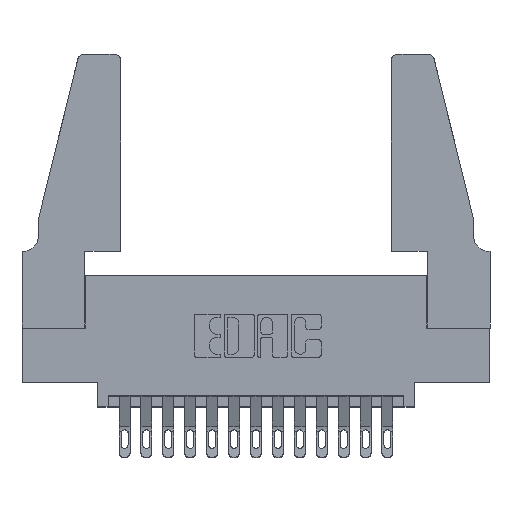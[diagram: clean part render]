
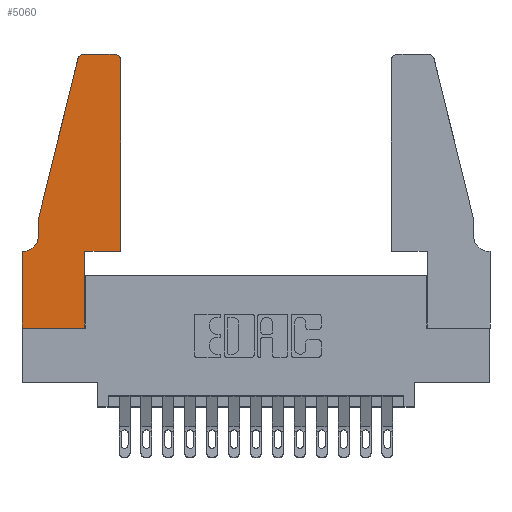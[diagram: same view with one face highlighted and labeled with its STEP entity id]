
A CAD part, top view. The second image highlights one B-rep face of the part: STEP entity #5060.
In plain terms, the highlighted planar face has unit normal (0, 0, 1).
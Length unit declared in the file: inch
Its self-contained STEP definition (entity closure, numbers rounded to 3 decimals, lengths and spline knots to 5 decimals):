
#208 = VECTOR ( 'NONE', #4959, 39.37008 ) ;
#373 = CARTESIAN_POINT ( 'NONE',  ( 0., 0., 0.37 ) ) ;
#740 = VERTEX_POINT ( 'NONE', #13154 ) ;
#792 = CARTESIAN_POINT ( 'NONE',  ( 0.0755, 0.5, 0.37 ) ) ;
#842 = EDGE_CURVE ( 'NONE', #12437, #2490, #10101, .T. ) ;
#954 = ORIENTED_EDGE ( 'NONE', *, *, #8056, .T. ) ;
#1024 = DIRECTION ( 'NONE',  ( 0., -1., 0. ) ) ;
#1128 = DIRECTION ( 'NONE',  ( 0., 0., 1. ) ) ;
#1302 = PLANE ( 'NONE',  #11525 ) ;
#1312 = VERTEX_POINT ( 'NONE', #3188 ) ;
#1723 = CARTESIAN_POINT ( 'NONE',  ( 0.0755, 0.5, 0.37 ) ) ;
#1902 = EDGE_CURVE ( 'NONE', #1312, #12437, #4942, .T. ) ;
#2243 = CARTESIAN_POINT ( 'NONE',  ( 0.0755, 0.35, 0.37 ) ) ;
#2398 = DIRECTION ( 'NONE',  ( 1., 0., 0. ) ) ;
#2412 = DIRECTION ( 'NONE',  ( 0., 1., 0. ) ) ;
#2463 = VERTEX_POINT ( 'NONE', #10306 ) ;
#2490 = VERTEX_POINT ( 'NONE', #11621 ) ;
#2513 = CARTESIAN_POINT ( 'NONE',  ( 0.4205, 1.25, 0.37 ) ) ;
#2810 = EDGE_CURVE ( 'NONE', #15947, #1312, #6769, .T. ) ;
#3042 = EDGE_CURVE ( 'NONE', #12901, #2463, #7192, .T. ) ;
#3188 = CARTESIAN_POINT ( 'NONE',  ( 0.284, 1.25, 0.37 ) ) ;
#3362 = EDGE_CURVE ( 'NONE', #10633, #10353, #14053, .T. ) ;
#3564 = CARTESIAN_POINT ( 'NONE',  ( 0., 0., 0.37 ) ) ;
#3699 = VECTOR ( 'NONE', #10752, 39.37008 ) ;
#3736 = ORIENTED_EDGE ( 'NONE', *, *, #15725, .T. ) ;
#3758 = ORIENTED_EDGE ( 'NONE', *, *, #3362, .T. ) ;
#4247 = VECTOR ( 'NONE', #8750, 39.37008 ) ;
#4432 = VECTOR ( 'NONE', #16582, 39.37008 ) ;
#4637 = ORIENTED_EDGE ( 'NONE', *, *, #842, .T. ) ;
#4734 = CARTESIAN_POINT ( 'NONE',  ( 0.0755, 0.42, 0.37 ) ) ;
#4803 = VERTEX_POINT ( 'NONE', #5946 ) ;
#4942 = CIRCLE ( 'NONE', #7488, 0.03 ) ;
#4943 = EDGE_CURVE ( 'NONE', #5863, #12901, #12502, .T. ) ;
#4959 = DIRECTION ( 'NONE',  ( 0., 1., 0. ) ) ;
#5060 = ADVANCED_FACE ( 'NONE', ( #13080 ), #1302, .T. ) ;
#5377 = CARTESIAN_POINT ( 'NONE',  ( 0.4505, 0.35, 0.37 ) ) ;
#5634 = AXIS2_PLACEMENT_3D ( 'NONE', #14523, #6773, #13348 ) ;
#5650 = ORIENTED_EDGE ( 'NONE', *, *, #2810, .T. ) ;
#5863 = VERTEX_POINT ( 'NONE', #13627 ) ;
#5946 = CARTESIAN_POINT ( 'NONE',  ( 0.4505, 1.22, 0.37 ) ) ;
#6074 = CARTESIAN_POINT ( 'NONE',  ( 0.4505, 0.35, 0.37 ) ) ;
#6419 = EDGE_LOOP ( 'NONE', ( #5650, #11657, #4637, #954, #3758, #13628, #7407, #14054, #10260, #3736, #7974, #16137 ) ) ;
#6554 = CIRCLE ( 'NONE', #16068, 0.03 ) ;
#6769 = LINE ( 'NONE', #16060, #8612 ) ;
#6773 = DIRECTION ( 'NONE',  ( 0., 0., -1. ) ) ;
#6912 = LINE ( 'NONE', #2243, #4247 ) ;
#7192 = LINE ( 'NONE', #8071, #3699 ) ;
#7333 = VECTOR ( 'NONE', #2412, 39.37008 ) ;
#7407 = ORIENTED_EDGE ( 'NONE', *, *, #4943, .T. ) ;
#7488 = AXIS2_PLACEMENT_3D ( 'NONE', #16594, #1128, #2398 ) ;
#7974 = ORIENTED_EDGE ( 'NONE', *, *, #15213, .T. ) ;
#8056 = EDGE_CURVE ( 'NONE', #2490, #10633, #15936, .T. ) ;
#8071 = CARTESIAN_POINT ( 'NONE',  ( 0., 0., 0.37 ) ) ;
#8483 = DIRECTION ( 'NONE',  ( -1., 0., 0. ) ) ;
#8612 = VECTOR ( 'NONE', #8483, 39.37008 ) ;
#8750 = DIRECTION ( 'NONE',  ( -1., 0., 0. ) ) ;
#9084 = CARTESIAN_POINT ( 'NONE',  ( 0.4505, 0.35, 0.37 ) ) ;
#9896 = CARTESIAN_POINT ( 'NONE',  ( 0.25487, 1.22718, 0.37 ) ) ;
#10022 = DIRECTION ( 'NONE',  ( 0., 0., 1. ) ) ;
#10101 = LINE ( 'NONE', #792, #11916 ) ;
#10182 = LINE ( 'NONE', #11493, #7333 ) ;
#10260 = ORIENTED_EDGE ( 'NONE', *, *, #15149, .T. ) ;
#10306 = CARTESIAN_POINT ( 'NONE',  ( 0.2865, 0., 0.37 ) ) ;
#10353 = VERTEX_POINT ( 'NONE', #10803 ) ;
#10390 = DIRECTION ( 'NONE',  ( 1., 0., 0. ) ) ;
#10633 = VERTEX_POINT ( 'NONE', #4734 ) ;
#10660 = VECTOR ( 'NONE', #1024, 39.37008 ) ;
#10752 = DIRECTION ( 'NONE',  ( 1., 0., 0. ) ) ;
#10803 = CARTESIAN_POINT ( 'NONE',  ( 0.0055, 0.35, 0.37 ) ) ;
#10945 = VERTEX_POINT ( 'NONE', #5377 ) ;
#11039 = DIRECTION ( 'NONE',  ( -0.239, -0.971, 0. ) ) ;
#11132 = DIRECTION ( 'NONE',  ( 1., 0., 0. ) ) ;
#11493 = CARTESIAN_POINT ( 'NONE',  ( 0.2865, 0.35, 0.37 ) ) ;
#11525 = AXIS2_PLACEMENT_3D ( 'NONE', #11594, #13993, #10390 ) ;
#11594 = CARTESIAN_POINT ( 'NONE',  ( 0., 0.35, 0.37 ) ) ;
#11621 = CARTESIAN_POINT ( 'NONE',  ( 0.0755, 0.5, 0.37 ) ) ;
#11657 = ORIENTED_EDGE ( 'NONE', *, *, #1902, .T. ) ;
#11916 = VECTOR ( 'NONE', #11039, 39.37008 ) ;
#12437 = VERTEX_POINT ( 'NONE', #9896 ) ;
#12502 = LINE ( 'NONE', #3564, #10660 ) ;
#12571 = CARTESIAN_POINT ( 'NONE',  ( 0.4205, 1.22, 0.37 ) ) ;
#12901 = VERTEX_POINT ( 'NONE', #373 ) ;
#13080 = FACE_OUTER_BOUND ( 'NONE', #6419, .T. ) ;
#13154 = CARTESIAN_POINT ( 'NONE',  ( 0.2865, 0.35, 0.37 ) ) ;
#13348 = DIRECTION ( 'NONE',  ( -1., 0., 0. ) ) ;
#13465 = DIRECTION ( 'NONE',  ( 0., -1., 0. ) ) ;
#13627 = CARTESIAN_POINT ( 'NONE',  ( 0., 0.35, 0.37 ) ) ;
#13628 = ORIENTED_EDGE ( 'NONE', *, *, #14987, .T. ) ;
#13741 = EDGE_CURVE ( 'NONE', #4803, #15947, #6554, .T. ) ;
#13993 = DIRECTION ( 'NONE',  ( 0., 0., 1. ) ) ;
#14053 = CIRCLE ( 'NONE', #5634, 0.07 ) ;
#14054 = ORIENTED_EDGE ( 'NONE', *, *, #3042, .T. ) ;
#14403 = LINE ( 'NONE', #6074, #4432 ) ;
#14523 = CARTESIAN_POINT ( 'NONE',  ( 0.0055, 0.42, 0.37 ) ) ;
#14604 = LINE ( 'NONE', #9084, #208 ) ;
#14987 = EDGE_CURVE ( 'NONE', #10353, #5863, #6912, .T. ) ;
#15149 = EDGE_CURVE ( 'NONE', #2463, #740, #10182, .T. ) ;
#15213 = EDGE_CURVE ( 'NONE', #10945, #4803, #14604, .T. ) ;
#15725 = EDGE_CURVE ( 'NONE', #740, #10945, #14403, .T. ) ;
#15936 = LINE ( 'NONE', #1723, #16529 ) ;
#15947 = VERTEX_POINT ( 'NONE', #2513 ) ;
#16060 = CARTESIAN_POINT ( 'NONE',  ( 0.2605, 1.25, 0.37 ) ) ;
#16068 = AXIS2_PLACEMENT_3D ( 'NONE', #12571, #10022, #11132 ) ;
#16137 = ORIENTED_EDGE ( 'NONE', *, *, #13741, .T. ) ;
#16529 = VECTOR ( 'NONE', #13465, 39.37008 ) ;
#16582 = DIRECTION ( 'NONE',  ( 1., 0., 0. ) ) ;
#16594 = CARTESIAN_POINT ( 'NONE',  ( 0.284, 1.22, 0.37 ) ) ;
